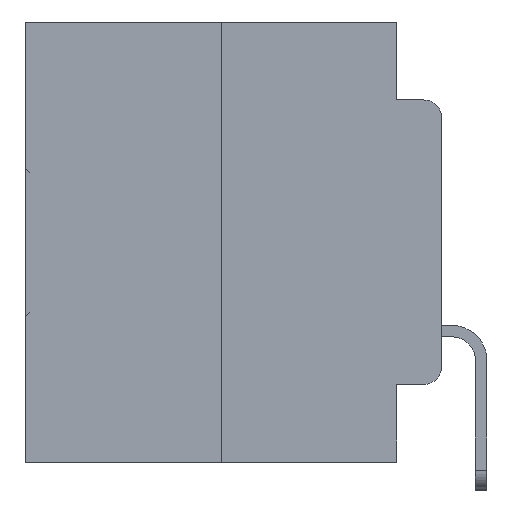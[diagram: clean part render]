
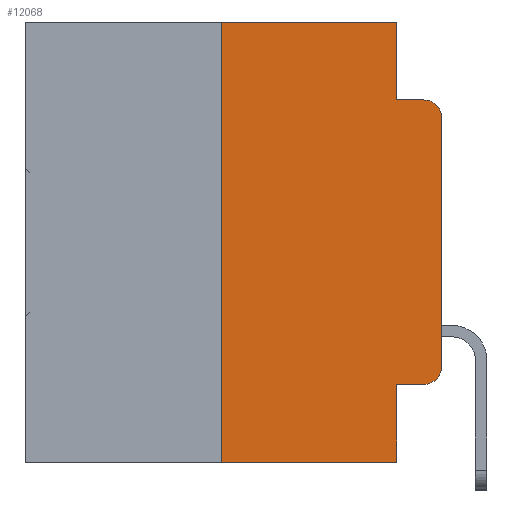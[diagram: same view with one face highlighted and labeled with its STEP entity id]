
A CAD part, left-side view. The second image highlights one B-rep face of the part: STEP entity #12068.
In plain terms, the highlighted planar face has unit normal (-1, 0, 0).
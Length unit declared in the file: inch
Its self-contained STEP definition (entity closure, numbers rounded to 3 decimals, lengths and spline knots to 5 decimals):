
#1379 = PLANE ( 'NONE',  #23409 ) ;
#1869 = EDGE_CURVE ( 'NONE', #18723, #27844, #29222, .T. ) ;
#1970 = DIRECTION ( 'NONE',  ( -1., 0., 0. ) ) ;
#1975 = CARTESIAN_POINT ( 'NONE',  ( 0., 0., 0. ) ) ;
#2164 = EDGE_CURVE ( 'NONE', #23684, #18062, #5784, .T. ) ;
#2834 = LINE ( 'NONE', #22831, #16134 ) ;
#3057 = ORIENTED_EDGE ( 'NONE', *, *, #21457, .F. ) ;
#3172 = EDGE_LOOP ( 'NONE', ( #29905, #28875, #30248, #16632, #27527, #19128, #4267, #3057, #5463, #21992 ) ) ;
#4267 = ORIENTED_EDGE ( 'NONE', *, *, #2164, .T. ) ;
#4500 = VERTEX_POINT ( 'NONE', #25141 ) ;
#4723 = LINE ( 'NONE', #5765, #11402 ) ;
#5463 = ORIENTED_EDGE ( 'NONE', *, *, #10386, .T. ) ;
#5765 = CARTESIAN_POINT ( 'NONE',  ( 0., 0.051, 0. ) ) ;
#5784 = LINE ( 'NONE', #7186, #6572 ) ;
#6572 = VECTOR ( 'NONE', #25978, 39.37008 ) ;
#7045 = LINE ( 'NONE', #29950, #12923 ) ;
#7050 = CARTESIAN_POINT ( 'NONE',  ( 0., 0.473, 0. ) ) ;
#7186 = CARTESIAN_POINT ( 'NONE',  ( 0., 0.473, -0.5 ) ) ;
#7443 = EDGE_CURVE ( 'NONE', #27844, #27958, #17111, .T. ) ;
#7964 = DIRECTION ( 'NONE',  ( -1., 0., 0. ) ) ;
#8157 = CIRCLE ( 'NONE', #13387, 0.02 ) ;
#8511 = CARTESIAN_POINT ( 'NONE',  ( 0., 0.25, 0. ) ) ;
#8704 = DIRECTION ( 'NONE',  ( 0., 0., 1. ) ) ;
#9041 = DIRECTION ( 'NONE',  ( 0., 0., -1. ) ) ;
#10386 = EDGE_CURVE ( 'NONE', #18446, #18723, #2834, .T. ) ;
#10994 = FACE_OUTER_BOUND ( 'NONE', #3172, .T. ) ;
#11074 = DIRECTION ( 'NONE',  ( 0., -1., 0. ) ) ;
#11402 = VECTOR ( 'NONE', #29181, 39.37008 ) ;
#11453 = EDGE_CURVE ( 'NONE', #14483, #4500, #4723, .T. ) ;
#11885 = LINE ( 'NONE', #29485, #17510 ) ;
#12068 = ADVANCED_FACE ( 'NONE', ( #10994 ), #1379, .F. ) ;
#12237 = VECTOR ( 'NONE', #16915, 39.37008 ) ;
#12923 = VECTOR ( 'NONE', #18931, 39.37008 ) ;
#13114 = EDGE_CURVE ( 'NONE', #4500, #24621, #29920, .T. ) ;
#13369 = CARTESIAN_POINT ( 'NONE',  ( 0., 0.051, -0.5 ) ) ;
#13387 = AXIS2_PLACEMENT_3D ( 'NONE', #16909, #1970, #19187 ) ;
#14032 = VECTOR ( 'NONE', #30416, 39.37008 ) ;
#14483 = VERTEX_POINT ( 'NONE', #19567 ) ;
#16134 = VECTOR ( 'NONE', #11074, 39.37008 ) ;
#16632 = ORIENTED_EDGE ( 'NONE', *, *, #11453, .F. ) ;
#16909 = CARTESIAN_POINT ( 'NONE',  ( 0., 0.02, -0.1085 ) ) ;
#16915 = DIRECTION ( 'NONE',  ( 0., 0., 1. ) ) ;
#17111 = LINE ( 'NONE', #1975, #12237 ) ;
#17510 = VECTOR ( 'NONE', #8704, 39.37008 ) ;
#17748 = AXIS2_PLACEMENT_3D ( 'NONE', #22221, #7964, #24447 ) ;
#17958 = CARTESIAN_POINT ( 'NONE',  ( 0., 0.051, -0.0885 ) ) ;
#18062 = VERTEX_POINT ( 'NONE', #13369 ) ;
#18129 = VERTEX_POINT ( 'NONE', #8511 ) ;
#18446 = VERTEX_POINT ( 'NONE', #27871 ) ;
#18503 = CARTESIAN_POINT ( 'NONE',  ( 0., 0.25, -0.5 ) ) ;
#18668 = CARTESIAN_POINT ( 'NONE',  ( 0., 0.473, 0. ) ) ;
#18723 = VERTEX_POINT ( 'NONE', #19659 ) ;
#18931 = DIRECTION ( 'NONE',  ( 0., 0., -1. ) ) ;
#19128 = ORIENTED_EDGE ( 'NONE', *, *, #30387, .F. ) ;
#19187 = DIRECTION ( 'NONE',  ( 0., 0., -1. ) ) ;
#19274 = CARTESIAN_POINT ( 'NONE',  ( 0., 0., -0.3915 ) ) ;
#19567 = CARTESIAN_POINT ( 'NONE',  ( 0., 0.051, 0. ) ) ;
#19659 = CARTESIAN_POINT ( 'NONE',  ( 0., 0.02, -0.4115 ) ) ;
#19664 = CARTESIAN_POINT ( 'NONE',  ( 0., 0., -0.1085 ) ) ;
#20159 = LINE ( 'NONE', #7050, #14032 ) ;
#21457 = EDGE_CURVE ( 'NONE', #18446, #18062, #7045, .T. ) ;
#21524 = CARTESIAN_POINT ( 'NONE',  ( 0., 0.02, -0.0885 ) ) ;
#21992 = ORIENTED_EDGE ( 'NONE', *, *, #1869, .T. ) ;
#22221 = CARTESIAN_POINT ( 'NONE',  ( 0., 0.02, -0.3915 ) ) ;
#22408 = EDGE_CURVE ( 'NONE', #27958, #24621, #8157, .T. ) ;
#22831 = CARTESIAN_POINT ( 'NONE',  ( 0., 0.051, -0.4115 ) ) ;
#23088 = EDGE_CURVE ( 'NONE', #18129, #14483, #20159, .T. ) ;
#23191 = DIRECTION ( 'NONE',  ( 1., 0., 0. ) ) ;
#23409 = AXIS2_PLACEMENT_3D ( 'NONE', #18668, #23191, #9041 ) ;
#23684 = VERTEX_POINT ( 'NONE', #18503 ) ;
#24014 = VECTOR ( 'NONE', #26969, 39.37008 ) ;
#24447 = DIRECTION ( 'NONE',  ( 0., 0., -1. ) ) ;
#24621 = VERTEX_POINT ( 'NONE', #21524 ) ;
#25141 = CARTESIAN_POINT ( 'NONE',  ( 0., 0.051, -0.0885 ) ) ;
#25978 = DIRECTION ( 'NONE',  ( 0., -1., 0. ) ) ;
#26969 = DIRECTION ( 'NONE',  ( 0., -1., 0. ) ) ;
#27527 = ORIENTED_EDGE ( 'NONE', *, *, #23088, .F. ) ;
#27844 = VERTEX_POINT ( 'NONE', #19274 ) ;
#27871 = CARTESIAN_POINT ( 'NONE',  ( 0., 0.051, -0.4115 ) ) ;
#27958 = VERTEX_POINT ( 'NONE', #19664 ) ;
#28875 = ORIENTED_EDGE ( 'NONE', *, *, #22408, .T. ) ;
#29181 = DIRECTION ( 'NONE',  ( 0., 0., -1. ) ) ;
#29222 = CIRCLE ( 'NONE', #17748, 0.02 ) ;
#29485 = CARTESIAN_POINT ( 'NONE',  ( 0., 0.25, 0. ) ) ;
#29905 = ORIENTED_EDGE ( 'NONE', *, *, #7443, .T. ) ;
#29920 = LINE ( 'NONE', #17958, #24014 ) ;
#29950 = CARTESIAN_POINT ( 'NONE',  ( 0., 0.051, 0. ) ) ;
#30248 = ORIENTED_EDGE ( 'NONE', *, *, #13114, .F. ) ;
#30387 = EDGE_CURVE ( 'NONE', #23684, #18129, #11885, .T. ) ;
#30416 = DIRECTION ( 'NONE',  ( 0., -1., 0. ) ) ;
